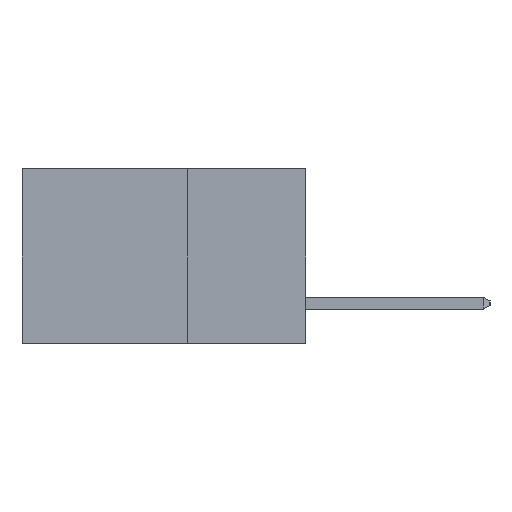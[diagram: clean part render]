
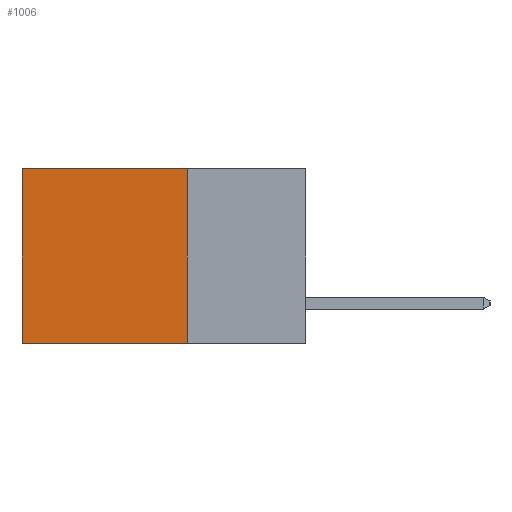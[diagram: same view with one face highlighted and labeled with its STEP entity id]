
A CAD part, left-side view. The second image highlights one B-rep face of the part: STEP entity #1006.
In plain terms, the highlighted planar face has unit normal (-1, 0, 0).
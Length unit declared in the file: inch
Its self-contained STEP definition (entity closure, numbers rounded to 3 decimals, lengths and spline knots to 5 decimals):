
#551 = VECTOR ( 'NONE', #9850, 39.37008 ) ;
#832 = DIRECTION ( 'NONE',  ( 0., 0., -1. ) ) ;
#1006 = ADVANCED_FACE ( 'NONE', ( #9533 ), #7680, .F. ) ;
#1496 = EDGE_CURVE ( 'NONE', #2915, #12444, #5976, .T. ) ;
#2721 = DIRECTION ( 'NONE',  ( 0., 1., 0. ) ) ;
#2915 = VERTEX_POINT ( 'NONE', #10439 ) ;
#3203 = EDGE_LOOP ( 'NONE', ( #8286, #4787, #3444, #3243 ) ) ;
#3243 = ORIENTED_EDGE ( 'NONE', *, *, #6560, .T. ) ;
#3323 = VECTOR ( 'NONE', #832, 39.37008 ) ;
#3444 = ORIENTED_EDGE ( 'NONE', *, *, #10036, .F. ) ;
#4787 = ORIENTED_EDGE ( 'NONE', *, *, #1496, .F. ) ;
#5105 = VERTEX_POINT ( 'NONE', #12637 ) ;
#5400 = LINE ( 'NONE', #10418, #12329 ) ;
#5760 = CARTESIAN_POINT ( 'NONE',  ( 0.2615, 0.6, -0.37 ) ) ;
#5976 = LINE ( 'NONE', #12306, #551 ) ;
#6560 = EDGE_CURVE ( 'NONE', #8052, #5105, #5400, .T. ) ;
#7355 = DIRECTION ( 'NONE',  ( 0., 0., -1. ) ) ;
#7680 = PLANE ( 'NONE',  #9983 ) ;
#7714 = CARTESIAN_POINT ( 'NONE',  ( 0.2615, 0.25, -0.37 ) ) ;
#7723 = DIRECTION ( 'NONE',  ( 1., 0., 0. ) ) ;
#8052 = VERTEX_POINT ( 'NONE', #10561 ) ;
#8286 = ORIENTED_EDGE ( 'NONE', *, *, #11352, .T. ) ;
#8492 = LINE ( 'NONE', #12452, #3323 ) ;
#9194 = VECTOR ( 'NONE', #10495, 39.37008 ) ;
#9476 = LINE ( 'NONE', #5760, #9194 ) ;
#9533 = FACE_OUTER_BOUND ( 'NONE', #3203, .T. ) ;
#9850 = DIRECTION ( 'NONE',  ( 0., 1., 0. ) ) ;
#9983 = AXIS2_PLACEMENT_3D ( 'NONE', #7714, #7723, #7355 ) ;
#10036 = EDGE_CURVE ( 'NONE', #8052, #2915, #8492, .T. ) ;
#10418 = CARTESIAN_POINT ( 'NONE',  ( 0.2615, 0.25, 0. ) ) ;
#10439 = CARTESIAN_POINT ( 'NONE',  ( 0.2615, 0.25, -0.37 ) ) ;
#10495 = DIRECTION ( 'NONE',  ( 0., 0., -1. ) ) ;
#10561 = CARTESIAN_POINT ( 'NONE',  ( 0.2615, 0.25, 0. ) ) ;
#11352 = EDGE_CURVE ( 'NONE', #5105, #12444, #9476, .T. ) ;
#11897 = CARTESIAN_POINT ( 'NONE',  ( 0.2615, 0.6, -0.37 ) ) ;
#12306 = CARTESIAN_POINT ( 'NONE',  ( 0.2615, 0.25, -0.37 ) ) ;
#12329 = VECTOR ( 'NONE', #2721, 39.37008 ) ;
#12444 = VERTEX_POINT ( 'NONE', #11897 ) ;
#12452 = CARTESIAN_POINT ( 'NONE',  ( 0.2615, 0.25, -0.37 ) ) ;
#12637 = CARTESIAN_POINT ( 'NONE',  ( 0.2615, 0.6, 0. ) ) ;
